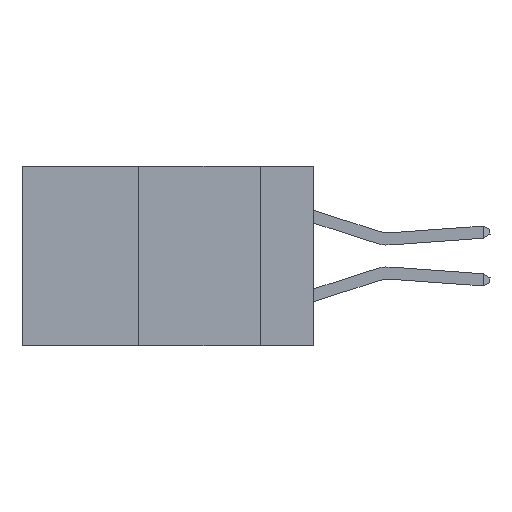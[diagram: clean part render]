
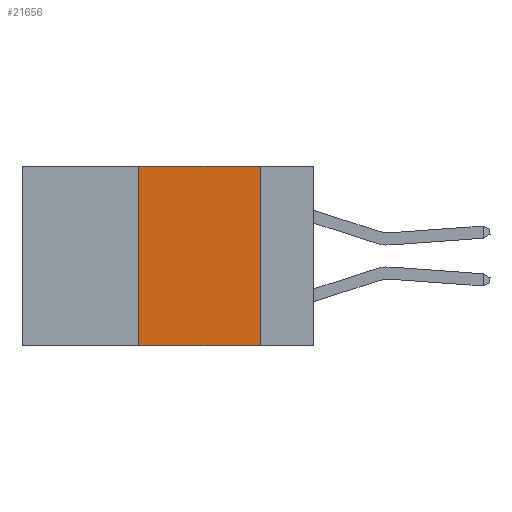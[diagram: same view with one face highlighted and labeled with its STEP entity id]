
A CAD part, left-side view. The second image highlights one B-rep face of the part: STEP entity #21656.
In plain terms, the highlighted planar face has unit normal (-1, 0, 0).
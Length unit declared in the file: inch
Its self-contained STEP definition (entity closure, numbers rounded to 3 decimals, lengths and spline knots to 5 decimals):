
#790 = DIRECTION ( 'NONE',  ( 0., 0., 1. ) ) ;
#1009 = DIRECTION ( 'NONE',  ( 0., 0., -1. ) ) ;
#1286 = CARTESIAN_POINT ( 'NONE',  ( 0., 0.6, 0. ) ) ;
#1963 = PLANE ( 'NONE',  #21604 ) ;
#1996 = ORIENTED_EDGE ( 'NONE', *, *, #16633, .F. ) ;
#3569 = CARTESIAN_POINT ( 'NONE',  ( 0., 0.11, 0. ) ) ;
#3604 = DIRECTION ( 'NONE',  ( 1., 0., 0. ) ) ;
#3827 = CARTESIAN_POINT ( 'NONE',  ( 0., 0.36, -0.37 ) ) ;
#3884 = DIRECTION ( 'NONE',  ( 0., 0., -1. ) ) ;
#4069 = VERTEX_POINT ( 'NONE', #3569 ) ;
#5122 = LINE ( 'NONE', #18751, #17865 ) ;
#5530 = EDGE_CURVE ( 'NONE', #19796, #5575, #11156, .T. ) ;
#5575 = VERTEX_POINT ( 'NONE', #6708 ) ;
#6708 = CARTESIAN_POINT ( 'NONE',  ( 0., 0.36, 0. ) ) ;
#6776 = DIRECTION ( 'NONE',  ( 0., -1., 0. ) ) ;
#11003 = VECTOR ( 'NONE', #17794, 39.37008 ) ;
#11156 = LINE ( 'NONE', #16026, #23364 ) ;
#11439 = ORIENTED_EDGE ( 'NONE', *, *, #12738, .T. ) ;
#11925 = EDGE_LOOP ( 'NONE', ( #1996, #18814, #18197, #11439 ) ) ;
#12738 = EDGE_CURVE ( 'NONE', #19796, #17686, #20349, .T. ) ;
#16026 = CARTESIAN_POINT ( 'NONE',  ( 0., 0.36, 0. ) ) ;
#16633 = EDGE_CURVE ( 'NONE', #4069, #17686, #5122, .T. ) ;
#17337 = EDGE_CURVE ( 'NONE', #5575, #4069, #20528, .T. ) ;
#17686 = VERTEX_POINT ( 'NONE', #18292 ) ;
#17794 = DIRECTION ( 'NONE',  ( 0., -1., 0. ) ) ;
#17865 = VECTOR ( 'NONE', #3884, 39.37008 ) ;
#18197 = ORIENTED_EDGE ( 'NONE', *, *, #5530, .F. ) ;
#18292 = CARTESIAN_POINT ( 'NONE',  ( 0., 0.11, -0.37 ) ) ;
#18751 = CARTESIAN_POINT ( 'NONE',  ( 0., 0.11, 0. ) ) ;
#18814 = ORIENTED_EDGE ( 'NONE', *, *, #17337, .F. ) ;
#19629 = CARTESIAN_POINT ( 'NONE',  ( 0., 0.6, 0. ) ) ;
#19796 = VERTEX_POINT ( 'NONE', #3827 ) ;
#20349 = LINE ( 'NONE', #22155, #22454 ) ;
#20528 = LINE ( 'NONE', #19629, #11003 ) ;
#21604 = AXIS2_PLACEMENT_3D ( 'NONE', #1286, #3604, #1009 ) ;
#21656 = ADVANCED_FACE ( 'NONE', ( #22717 ), #1963, .F. ) ;
#22155 = CARTESIAN_POINT ( 'NONE',  ( 0., 0.6, -0.37 ) ) ;
#22454 = VECTOR ( 'NONE', #6776, 39.37008 ) ;
#22717 = FACE_OUTER_BOUND ( 'NONE', #11925, .T. ) ;
#23364 = VECTOR ( 'NONE', #790, 39.37008 ) ;
